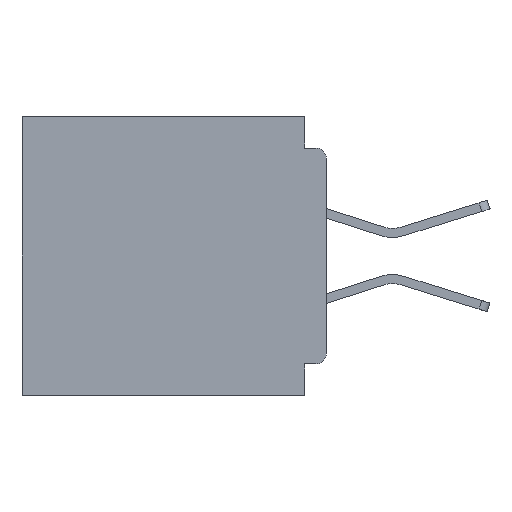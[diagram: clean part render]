
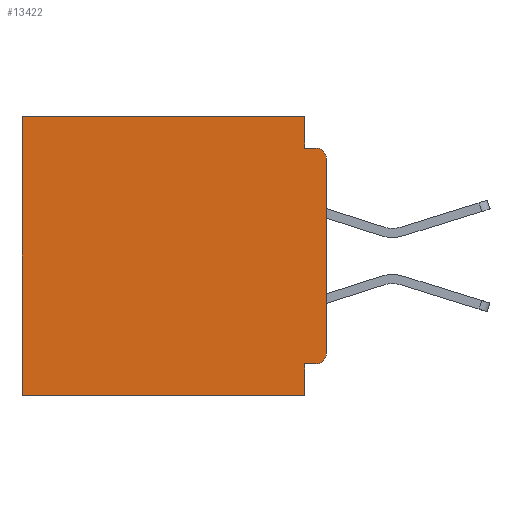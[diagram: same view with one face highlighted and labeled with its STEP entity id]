
A CAD part, left-side view. The second image highlights one B-rep face of the part: STEP entity #13422.
In plain terms, the highlighted planar face has unit normal (-1, 0, 0).
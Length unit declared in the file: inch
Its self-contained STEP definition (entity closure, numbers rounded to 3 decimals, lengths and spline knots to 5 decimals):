
#633 = CARTESIAN_POINT ( 'NONE',  ( 0.3, 0., -0.045 ) ) ;
#985 = DIRECTION ( 'NONE',  ( 0., 0., -1. ) ) ;
#1606 = VERTEX_POINT ( 'NONE', #6396 ) ;
#1958 = VECTOR ( 'NONE', #20241, 39.37008 ) ;
#2333 = ORIENTED_EDGE ( 'NONE', *, *, #32577, .T. ) ;
#2703 = LINE ( 'NONE', #633, #17410 ) ;
#4380 = DIRECTION ( 'NONE',  ( 0., 1., 0. ) ) ;
#4635 = CARTESIAN_POINT ( 'NONE',  ( 0.3, 0., -0.4 ) ) ;
#4708 = EDGE_CURVE ( 'NONE', #5489, #21627, #10685, .T. ) ;
#5000 = VECTOR ( 'NONE', #11118, 39.37008 ) ;
#5489 = VERTEX_POINT ( 'NONE', #14995 ) ;
#5692 = CARTESIAN_POINT ( 'NONE',  ( 0.3, 0.015, -0.06 ) ) ;
#6396 = CARTESIAN_POINT ( 'NONE',  ( 0.3, 0.437, 0. ) ) ;
#6469 = PLANE ( 'NONE',  #16449 ) ;
#6699 = VERTEX_POINT ( 'NONE', #36153 ) ;
#7322 = VERTEX_POINT ( 'NONE', #33739 ) ;
#7462 = VERTEX_POINT ( 'NONE', #34494 ) ;
#7531 = DIRECTION ( 'NONE',  ( 0., 0., -1. ) ) ;
#7720 = EDGE_CURVE ( 'NONE', #18071, #6699, #2703, .T. ) ;
#8626 = DIRECTION ( 'NONE',  ( 0., 0., -1. ) ) ;
#8738 = ORIENTED_EDGE ( 'NONE', *, *, #23068, .F. ) ;
#9511 = CARTESIAN_POINT ( 'NONE',  ( 0.3, 0.031, 0. ) ) ;
#9513 = CARTESIAN_POINT ( 'NONE',  ( 0.3, 0., -0.34 ) ) ;
#9674 = EDGE_CURVE ( 'NONE', #7462, #33936, #37140, .T. ) ;
#10504 = LINE ( 'NONE', #19011, #17407 ) ;
#10685 = LINE ( 'NONE', #25926, #1958 ) ;
#11011 = CARTESIAN_POINT ( 'NONE',  ( 0.3, 0.031, -0.355 ) ) ;
#11084 = VERTEX_POINT ( 'NONE', #24776 ) ;
#11118 = DIRECTION ( 'NONE',  ( 0., 1., 0. ) ) ;
#12332 = DIRECTION ( 'NONE',  ( 1., 0., 0. ) ) ;
#12431 = ORIENTED_EDGE ( 'NONE', *, *, #18051, .F. ) ;
#12875 = VECTOR ( 'NONE', #7531, 39.37008 ) ;
#13422 = ADVANCED_FACE ( 'NONE', ( #35988 ), #6469, .F. ) ;
#14029 = VECTOR ( 'NONE', #19533, 39.37008 ) ;
#14357 = VECTOR ( 'NONE', #27273, 39.37008 ) ;
#14963 = LINE ( 'NONE', #33933, #14029 ) ;
#14995 = CARTESIAN_POINT ( 'NONE',  ( 0.3, 0.015, -0.355 ) ) ;
#15535 = CIRCLE ( 'NONE', #26711, 0.015 ) ;
#16449 = AXIS2_PLACEMENT_3D ( 'NONE', #27025, #12332, #32755 ) ;
#16833 = EDGE_CURVE ( 'NONE', #7462, #6699, #15535, .T. ) ;
#17407 = VECTOR ( 'NONE', #4380, 39.37008 ) ;
#17410 = VECTOR ( 'NONE', #18106, 39.37008 ) ;
#18051 = EDGE_CURVE ( 'NONE', #7322, #19786, #27507, .T. ) ;
#18071 = VERTEX_POINT ( 'NONE', #20028 ) ;
#18106 = DIRECTION ( 'NONE',  ( 0., -1., 0. ) ) ;
#18393 = ORIENTED_EDGE ( 'NONE', *, *, #21535, .T. ) ;
#18593 = DIRECTION ( 'NONE',  ( -1., 0., 0. ) ) ;
#19011 = CARTESIAN_POINT ( 'NONE',  ( 0.3, 0., 0. ) ) ;
#19406 = DIRECTION ( 'NONE',  ( 0., 0., -1. ) ) ;
#19533 = DIRECTION ( 'NONE',  ( 0., 0., -1. ) ) ;
#19786 = VERTEX_POINT ( 'NONE', #23042 ) ;
#20028 = CARTESIAN_POINT ( 'NONE',  ( 0.3, 0.031, -0.045 ) ) ;
#20226 = EDGE_LOOP ( 'NONE', ( #20712, #34691, #29394, #8738, #23544, #18393, #12431, #29876, #23107, #2333 ) ) ;
#20241 = DIRECTION ( 'NONE',  ( 0., 1., 0. ) ) ;
#20712 = ORIENTED_EDGE ( 'NONE', *, *, #9674, .F. ) ;
#21535 = EDGE_CURVE ( 'NONE', #1606, #19786, #14963, .T. ) ;
#21627 = VERTEX_POINT ( 'NONE', #11011 ) ;
#22254 = CARTESIAN_POINT ( 'NONE',  ( 0.3, 0.031, -0.4 ) ) ;
#22326 = LINE ( 'NONE', #9511, #14357 ) ;
#23042 = CARTESIAN_POINT ( 'NONE',  ( 0.3, 0.437, -0.4 ) ) ;
#23068 = EDGE_CURVE ( 'NONE', #11084, #18071, #22326, .T. ) ;
#23107 = ORIENTED_EDGE ( 'NONE', *, *, #4708, .F. ) ;
#23544 = ORIENTED_EDGE ( 'NONE', *, *, #26400, .T. ) ;
#23573 = CIRCLE ( 'NONE', #24080, 0.015 ) ;
#24080 = AXIS2_PLACEMENT_3D ( 'NONE', #35902, #18593, #985 ) ;
#24776 = CARTESIAN_POINT ( 'NONE',  ( 0.3, 0.031, 0. ) ) ;
#25329 = EDGE_CURVE ( 'NONE', #21627, #7322, #27635, .T. ) ;
#25926 = CARTESIAN_POINT ( 'NONE',  ( 0.3, 0., -0.355 ) ) ;
#26286 = DIRECTION ( 'NONE',  ( -1., 0., 0. ) ) ;
#26400 = EDGE_CURVE ( 'NONE', #11084, #1606, #10504, .T. ) ;
#26711 = AXIS2_PLACEMENT_3D ( 'NONE', #5692, #26286, #8626 ) ;
#27025 = CARTESIAN_POINT ( 'NONE',  ( 0.3, 0., -0.4 ) ) ;
#27273 = DIRECTION ( 'NONE',  ( 0., 0., -1. ) ) ;
#27507 = LINE ( 'NONE', #31566, #5000 ) ;
#27635 = LINE ( 'NONE', #22254, #12875 ) ;
#27810 = VECTOR ( 'NONE', #19406, 39.37008 ) ;
#29394 = ORIENTED_EDGE ( 'NONE', *, *, #7720, .F. ) ;
#29876 = ORIENTED_EDGE ( 'NONE', *, *, #25329, .F. ) ;
#31566 = CARTESIAN_POINT ( 'NONE',  ( 0.3, 0., -0.4 ) ) ;
#32577 = EDGE_CURVE ( 'NONE', #5489, #33936, #23573, .T. ) ;
#32755 = DIRECTION ( 'NONE',  ( 0., 0., -1. ) ) ;
#33739 = CARTESIAN_POINT ( 'NONE',  ( 0.3, 0.031, -0.4 ) ) ;
#33933 = CARTESIAN_POINT ( 'NONE',  ( 0.3, 0.437, -0.4 ) ) ;
#33936 = VERTEX_POINT ( 'NONE', #9513 ) ;
#34494 = CARTESIAN_POINT ( 'NONE',  ( 0.3, 0., -0.06 ) ) ;
#34691 = ORIENTED_EDGE ( 'NONE', *, *, #16833, .T. ) ;
#35902 = CARTESIAN_POINT ( 'NONE',  ( 0.3, 0.015, -0.34 ) ) ;
#35988 = FACE_OUTER_BOUND ( 'NONE', #20226, .T. ) ;
#36153 = CARTESIAN_POINT ( 'NONE',  ( 0.3, 0.015, -0.045 ) ) ;
#37140 = LINE ( 'NONE', #4635, #27810 ) ;
